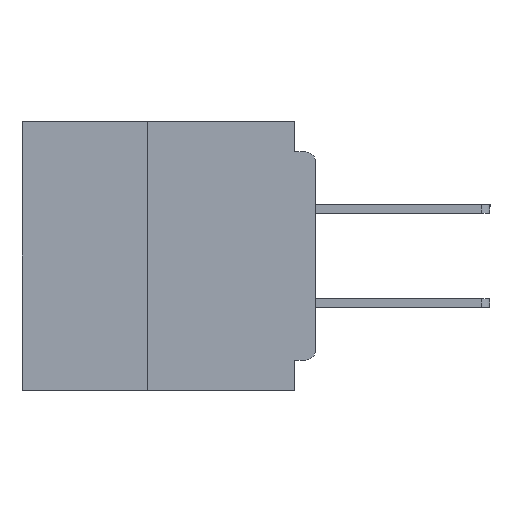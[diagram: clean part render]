
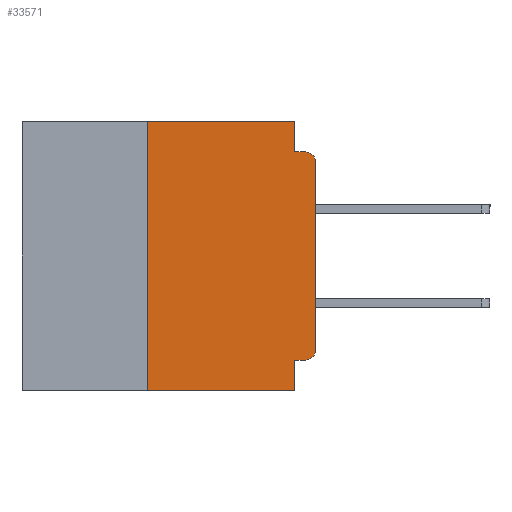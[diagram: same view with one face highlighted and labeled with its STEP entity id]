
A CAD part, left-side view. The second image highlights one B-rep face of the part: STEP entity #33571.
In plain terms, the highlighted planar face has unit normal (-1, 0, 0).
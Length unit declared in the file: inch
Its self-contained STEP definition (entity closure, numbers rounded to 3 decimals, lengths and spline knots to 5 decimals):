
#315 = CARTESIAN_POINT ( 'NONE',  ( 0., 0.015, -0.355 ) ) ;
#612 = CARTESIAN_POINT ( 'NONE',  ( 0., 0.25, 0. ) ) ;
#764 = CARTESIAN_POINT ( 'NONE',  ( 0., 0., -0.045 ) ) ;
#1448 = ORIENTED_EDGE ( 'NONE', *, *, #13324, .F. ) ;
#5225 = DIRECTION ( 'NONE',  ( 0., 0., 1. ) ) ;
#5470 = AXIS2_PLACEMENT_3D ( 'NONE', #56129, #23680, #61573 ) ;
#5974 = ORIENTED_EDGE ( 'NONE', *, *, #45966, .T. ) ;
#6612 = CARTESIAN_POINT ( 'NONE',  ( 0., 0.015, -0.06 ) ) ;
#9430 = LINE ( 'NONE', #32389, #35011 ) ;
#9682 = CARTESIAN_POINT ( 'NONE',  ( 0., 0.031, -0.4 ) ) ;
#10729 = EDGE_CURVE ( 'NONE', #50800, #69263, #69389, .T. ) ;
#11032 = EDGE_CURVE ( 'NONE', #35024, #14400, #36486, .T. ) ;
#12067 = DIRECTION ( 'NONE',  ( 0., 0., -1. ) ) ;
#12222 = CARTESIAN_POINT ( 'NONE',  ( 0., 0., 0. ) ) ;
#13324 = EDGE_CURVE ( 'NONE', #25919, #35024, #57334, .T. ) ;
#14400 = VERTEX_POINT ( 'NONE', #62843 ) ;
#14461 = VERTEX_POINT ( 'NONE', #47241 ) ;
#14611 = ORIENTED_EDGE ( 'NONE', *, *, #11032, .F. ) ;
#14681 = DIRECTION ( 'NONE',  ( 1., 0., 0. ) ) ;
#15613 = CARTESIAN_POINT ( 'NONE',  ( 0., 0., -0.06 ) ) ;
#15680 = EDGE_LOOP ( 'NONE', ( #66218, #67693, #32014, #14611, #1448, #55120, #5974, #44427, #51857, #59087 ) ) ;
#16616 = DIRECTION ( 'NONE',  ( 0., -1., 0. ) ) ;
#16885 = VECTOR ( 'NONE', #42245, 39.37008 ) ;
#17679 = DIRECTION ( 'NONE',  ( 0., 0., 1. ) ) ;
#20434 = EDGE_CURVE ( 'NONE', #14461, #40358, #45791, .T. ) ;
#22132 = CARTESIAN_POINT ( 'NONE',  ( 0., 0.031, -0.4 ) ) ;
#23043 = CARTESIAN_POINT ( 'NONE',  ( 0., 0.015, -0.045 ) ) ;
#23680 = DIRECTION ( 'NONE',  ( -1., 0., 0. ) ) ;
#24603 = DIRECTION ( 'NONE',  ( 0., 1., 0. ) ) ;
#25368 = VECTOR ( 'NONE', #31040, 39.37008 ) ;
#25507 = CARTESIAN_POINT ( 'NONE',  ( 0., 0.031, 0. ) ) ;
#25919 = VERTEX_POINT ( 'NONE', #612 ) ;
#26263 = VECTOR ( 'NONE', #17679, 39.37008 ) ;
#28164 = CARTESIAN_POINT ( 'NONE',  ( 0., 0.25, -0.4 ) ) ;
#30764 = CARTESIAN_POINT ( 'NONE',  ( 0., 0.437, 0. ) ) ;
#31040 = DIRECTION ( 'NONE',  ( 0., 0., -1. ) ) ;
#32014 = ORIENTED_EDGE ( 'NONE', *, *, #35905, .F. ) ;
#32389 = CARTESIAN_POINT ( 'NONE',  ( 0., 0.25, -0.4 ) ) ;
#32599 = VERTEX_POINT ( 'NONE', #315 ) ;
#32663 = VERTEX_POINT ( 'NONE', #28164 ) ;
#33571 = ADVANCED_FACE ( 'NONE', ( #43669 ), #41809, .F. ) ;
#34162 = LINE ( 'NONE', #764, #46790 ) ;
#35011 = VECTOR ( 'NONE', #5225, 39.37008 ) ;
#35024 = VERTEX_POINT ( 'NONE', #36591 ) ;
#35905 = EDGE_CURVE ( 'NONE', #14400, #37504, #34162, .T. ) ;
#36486 = LINE ( 'NONE', #25507, #25368 ) ;
#36591 = CARTESIAN_POINT ( 'NONE',  ( 0., 0.031, 0. ) ) ;
#37504 = VERTEX_POINT ( 'NONE', #23043 ) ;
#38343 = CARTESIAN_POINT ( 'NONE',  ( 0., 0.437, -0.4 ) ) ;
#39565 = LINE ( 'NONE', #67887, #53862 ) ;
#39753 = CIRCLE ( 'NONE', #5470, 0.015 ) ;
#40358 = VERTEX_POINT ( 'NONE', #22132 ) ;
#41809 = PLANE ( 'NONE',  #59123 ) ;
#42245 = DIRECTION ( 'NONE',  ( 0., 0., -1. ) ) ;
#43669 = FACE_OUTER_BOUND ( 'NONE', #15680, .T. ) ;
#44427 = ORIENTED_EDGE ( 'NONE', *, *, #20434, .F. ) ;
#44618 = DIRECTION ( 'NONE',  ( -1., 0., 0. ) ) ;
#44834 = EDGE_CURVE ( 'NONE', #32599, #50800, #39753, .T. ) ;
#45791 = LINE ( 'NONE', #9682, #16885 ) ;
#45966 = EDGE_CURVE ( 'NONE', #32663, #40358, #64055, .T. ) ;
#46790 = VECTOR ( 'NONE', #60511, 39.37008 ) ;
#47241 = CARTESIAN_POINT ( 'NONE',  ( 0., 0.031, -0.355 ) ) ;
#48859 = CIRCLE ( 'NONE', #55521, 0.015 ) ;
#50435 = CARTESIAN_POINT ( 'NONE',  ( 0., 0., -0.34 ) ) ;
#50800 = VERTEX_POINT ( 'NONE', #50435 ) ;
#51857 = ORIENTED_EDGE ( 'NONE', *, *, #61694, .F. ) ;
#52621 = DIRECTION ( 'NONE',  ( 0., 0., -1. ) ) ;
#53862 = VECTOR ( 'NONE', #24603, 39.37008 ) ;
#55120 = ORIENTED_EDGE ( 'NONE', *, *, #57568, .F. ) ;
#55521 = AXIS2_PLACEMENT_3D ( 'NONE', #6612, #44618, #12067 ) ;
#56129 = CARTESIAN_POINT ( 'NONE',  ( 0., 0.015, -0.34 ) ) ;
#57334 = LINE ( 'NONE', #30764, #69950 ) ;
#57568 = EDGE_CURVE ( 'NONE', #32663, #25919, #9430, .T. ) ;
#59087 = ORIENTED_EDGE ( 'NONE', *, *, #44834, .T. ) ;
#59123 = AXIS2_PLACEMENT_3D ( 'NONE', #68436, #14681, #52621 ) ;
#60511 = DIRECTION ( 'NONE',  ( 0., -1., 0. ) ) ;
#61573 = DIRECTION ( 'NONE',  ( 0., 0., -1. ) ) ;
#61694 = EDGE_CURVE ( 'NONE', #32599, #14461, #39565, .T. ) ;
#62843 = CARTESIAN_POINT ( 'NONE',  ( 0., 0.031, -0.045 ) ) ;
#63339 = DIRECTION ( 'NONE',  ( 0., -1., 0. ) ) ;
#64055 = LINE ( 'NONE', #38343, #65743 ) ;
#64772 = EDGE_CURVE ( 'NONE', #69263, #37504, #48859, .T. ) ;
#65743 = VECTOR ( 'NONE', #16616, 39.37008 ) ;
#66218 = ORIENTED_EDGE ( 'NONE', *, *, #10729, .T. ) ;
#67693 = ORIENTED_EDGE ( 'NONE', *, *, #64772, .T. ) ;
#67887 = CARTESIAN_POINT ( 'NONE',  ( 0., 0., -0.355 ) ) ;
#68436 = CARTESIAN_POINT ( 'NONE',  ( 0., 0.437, 0. ) ) ;
#69263 = VERTEX_POINT ( 'NONE', #15613 ) ;
#69389 = LINE ( 'NONE', #12222, #26263 ) ;
#69950 = VECTOR ( 'NONE', #63339, 39.37008 ) ;
